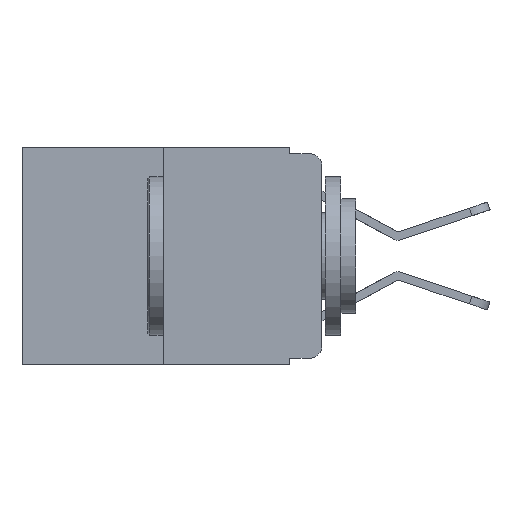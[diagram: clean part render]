
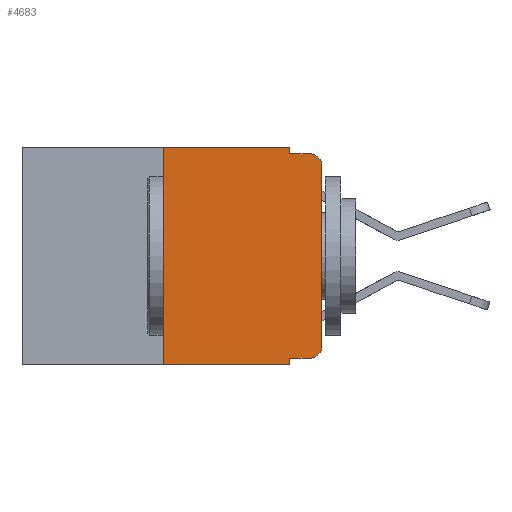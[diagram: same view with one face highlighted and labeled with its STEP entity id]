
A CAD part, left-side view. The second image highlights one B-rep face of the part: STEP entity #4683.
In plain terms, the highlighted planar face has unit normal (-1, 0, 0).
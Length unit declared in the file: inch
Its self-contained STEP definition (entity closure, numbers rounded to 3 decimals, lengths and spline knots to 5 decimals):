
#50 = VECTOR ( 'NONE', #3677, 39.37008 ) ;
#59 = EDGE_CURVE ( 'NONE', #13256, #6883, #11626, .T. ) ;
#372 = CIRCLE ( 'NONE', #1305, 0.02 ) ;
#396 = VERTEX_POINT ( 'NONE', #12522 ) ;
#599 = ORIENTED_EDGE ( 'NONE', *, *, #59, .T. ) ;
#934 = CARTESIAN_POINT ( 'NONE',  ( 0., 0.02, -0.03 ) ) ;
#994 = EDGE_CURVE ( 'NONE', #7860, #13256, #12530, .T. ) ;
#1033 = ORIENTED_EDGE ( 'NONE', *, *, #11518, .F. ) ;
#1230 = CARTESIAN_POINT ( 'NONE',  ( 0., 0.051, -0.01 ) ) ;
#1305 = AXIS2_PLACEMENT_3D ( 'NONE', #1413, #9236, #2681 ) ;
#1315 = CARTESIAN_POINT ( 'NONE',  ( 0., 0.051, -0.01 ) ) ;
#1413 = CARTESIAN_POINT ( 'NONE',  ( 0., 0.02, -0.313 ) ) ;
#1438 = VERTEX_POINT ( 'NONE', #1315 ) ;
#1575 = VECTOR ( 'NONE', #11914, 39.37008 ) ;
#1652 = ORIENTED_EDGE ( 'NONE', *, *, #12852, .F. ) ;
#2150 = CARTESIAN_POINT ( 'NONE',  ( 0., 0., -0.03 ) ) ;
#2424 = DIRECTION ( 'NONE',  ( 1., 0., 0. ) ) ;
#2681 = DIRECTION ( 'NONE',  ( 0., 0., -1. ) ) ;
#2847 = CARTESIAN_POINT ( 'NONE',  ( 0., 0.473, -0.343 ) ) ;
#3131 = CARTESIAN_POINT ( 'NONE',  ( 0., 0.25, 0. ) ) ;
#3185 = EDGE_CURVE ( 'NONE', #5195, #7896, #14087, .T. ) ;
#3282 = CARTESIAN_POINT ( 'NONE',  ( 0., 0.051, 0. ) ) ;
#3521 = ORIENTED_EDGE ( 'NONE', *, *, #994, .T. ) ;
#3677 = DIRECTION ( 'NONE',  ( 0., 0., -1. ) ) ;
#4194 = DIRECTION ( 'NONE',  ( 0., 0., 1. ) ) ;
#4222 = ORIENTED_EDGE ( 'NONE', *, *, #10862, .T. ) ;
#4568 = VERTEX_POINT ( 'NONE', #3282 ) ;
#4608 = CARTESIAN_POINT ( 'NONE',  ( 0., 0., 0. ) ) ;
#4650 = LINE ( 'NONE', #13873, #1575 ) ;
#4683 = ADVANCED_FACE ( 'NONE', ( #6405 ), #13946, .F. ) ;
#5195 = VERTEX_POINT ( 'NONE', #13367 ) ;
#5684 = VECTOR ( 'NONE', #12536, 39.37008 ) ;
#6034 = EDGE_LOOP ( 'NONE', ( #3521, #599, #9769, #1652, #8987, #9312, #9621, #1033, #4222, #12561 ) ) ;
#6345 = VECTOR ( 'NONE', #8035, 39.37008 ) ;
#6368 = CARTESIAN_POINT ( 'NONE',  ( 0., 0.25, 0. ) ) ;
#6384 = CARTESIAN_POINT ( 'NONE',  ( 0., 0.473, 0. ) ) ;
#6405 = FACE_OUTER_BOUND ( 'NONE', #6034, .T. ) ;
#6883 = VERTEX_POINT ( 'NONE', #10850 ) ;
#7136 = CARTESIAN_POINT ( 'NONE',  ( 0., 0.051, -0.333 ) ) ;
#7495 = VERTEX_POINT ( 'NONE', #8113 ) ;
#7847 = VERTEX_POINT ( 'NONE', #3131 ) ;
#7860 = VERTEX_POINT ( 'NONE', #11605 ) ;
#7896 = VERTEX_POINT ( 'NONE', #10660 ) ;
#7958 = LINE ( 'NONE', #7136, #9728 ) ;
#8035 = DIRECTION ( 'NONE',  ( 0., -1., 0. ) ) ;
#8113 = CARTESIAN_POINT ( 'NONE',  ( 0., 0.051, -0.333 ) ) ;
#8221 = DIRECTION ( 'NONE',  ( 0., -1., 0. ) ) ;
#8987 = ORIENTED_EDGE ( 'NONE', *, *, #14103, .F. ) ;
#9006 = CARTESIAN_POINT ( 'NONE',  ( 0., 0.473, 0. ) ) ;
#9068 = LINE ( 'NONE', #1230, #6345 ) ;
#9236 = DIRECTION ( 'NONE',  ( -1., 0., 0. ) ) ;
#9312 = ORIENTED_EDGE ( 'NONE', *, *, #12193, .F. ) ;
#9610 = DIRECTION ( 'NONE',  ( 0., -1., 0. ) ) ;
#9621 = ORIENTED_EDGE ( 'NONE', *, *, #3185, .T. ) ;
#9691 = VECTOR ( 'NONE', #9610, 39.37008 ) ;
#9728 = VECTOR ( 'NONE', #8221, 39.37008 ) ;
#9769 = ORIENTED_EDGE ( 'NONE', *, *, #13537, .F. ) ;
#9887 = VECTOR ( 'NONE', #4194, 39.37008 ) ;
#9987 = LINE ( 'NONE', #6384, #9691 ) ;
#9999 = DIRECTION ( 'NONE',  ( 0., 0., -1. ) ) ;
#10087 = CARTESIAN_POINT ( 'NONE',  ( 0., 0.051, 0. ) ) ;
#10201 = EDGE_CURVE ( 'NONE', #396, #7860, #372, .T. ) ;
#10376 = DIRECTION ( 'NONE',  ( 0., -1., 0. ) ) ;
#10660 = CARTESIAN_POINT ( 'NONE',  ( 0., 0.051, -0.343 ) ) ;
#10833 = VECTOR ( 'NONE', #10376, 39.37008 ) ;
#10850 = CARTESIAN_POINT ( 'NONE',  ( 0., 0.02, -0.01 ) ) ;
#10862 = EDGE_CURVE ( 'NONE', #7495, #396, #7958, .T. ) ;
#10929 = LINE ( 'NONE', #6368, #5684 ) ;
#11491 = DIRECTION ( 'NONE',  ( 0., 0., -1. ) ) ;
#11518 = EDGE_CURVE ( 'NONE', #7495, #7896, #4650, .T. ) ;
#11605 = CARTESIAN_POINT ( 'NONE',  ( 0., 0., -0.313 ) ) ;
#11626 = CIRCLE ( 'NONE', #13336, 0.02 ) ;
#11837 = LINE ( 'NONE', #10087, #50 ) ;
#11914 = DIRECTION ( 'NONE',  ( 0., 0., -1. ) ) ;
#12193 = EDGE_CURVE ( 'NONE', #5195, #7847, #10929, .T. ) ;
#12467 = DIRECTION ( 'NONE',  ( -1., 0., 0. ) ) ;
#12522 = CARTESIAN_POINT ( 'NONE',  ( 0., 0.02, -0.333 ) ) ;
#12530 = LINE ( 'NONE', #4608, #9887 ) ;
#12536 = DIRECTION ( 'NONE',  ( 0., 0., 1. ) ) ;
#12561 = ORIENTED_EDGE ( 'NONE', *, *, #10201, .T. ) ;
#12852 = EDGE_CURVE ( 'NONE', #4568, #1438, #11837, .T. ) ;
#13055 = AXIS2_PLACEMENT_3D ( 'NONE', #9006, #2424, #9999 ) ;
#13256 = VERTEX_POINT ( 'NONE', #2150 ) ;
#13336 = AXIS2_PLACEMENT_3D ( 'NONE', #934, #12467, #11491 ) ;
#13367 = CARTESIAN_POINT ( 'NONE',  ( 0., 0.25, -0.343 ) ) ;
#13537 = EDGE_CURVE ( 'NONE', #1438, #6883, #9068, .T. ) ;
#13873 = CARTESIAN_POINT ( 'NONE',  ( 0., 0.051, 0. ) ) ;
#13946 = PLANE ( 'NONE',  #13055 ) ;
#14087 = LINE ( 'NONE', #2847, #10833 ) ;
#14103 = EDGE_CURVE ( 'NONE', #7847, #4568, #9987, .T. ) ;
